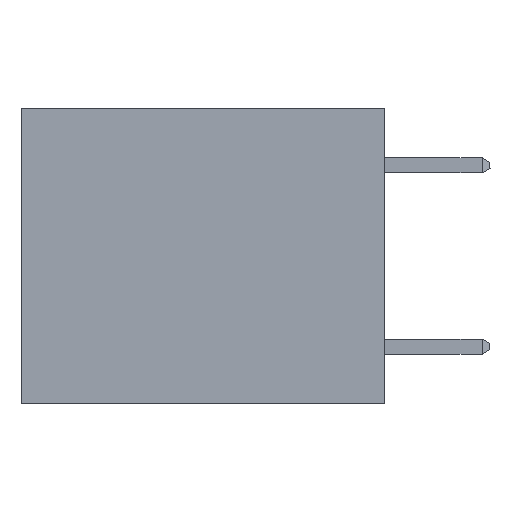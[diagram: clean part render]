
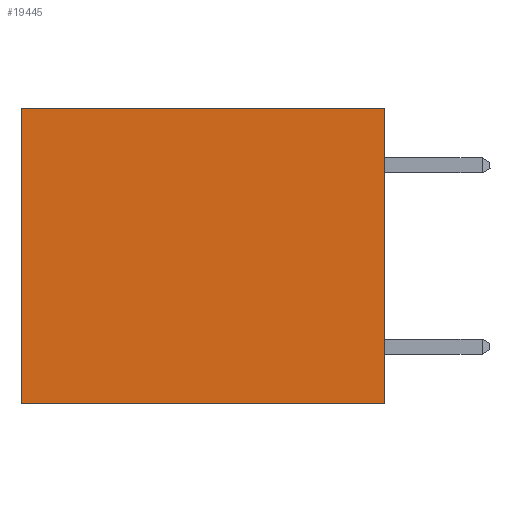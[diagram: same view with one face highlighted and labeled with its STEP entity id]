
A CAD part, left-side view. The second image highlights one B-rep face of the part: STEP entity #19445.
In plain terms, the highlighted planar face has unit normal (-1, 0, 0).
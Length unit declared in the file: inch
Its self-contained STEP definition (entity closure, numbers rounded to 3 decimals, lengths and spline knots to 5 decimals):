
#805 = VERTEX_POINT ( 'NONE', #16092 ) ;
#4127 = EDGE_CURVE ( 'NONE', #5492, #805, #22558, .T. ) ;
#5492 = VERTEX_POINT ( 'NONE', #27731 ) ;
#6005 = CARTESIAN_POINT ( 'NONE',  ( 0.3165, 0., -0.49 ) ) ;
#8502 = ORIENTED_EDGE ( 'NONE', *, *, #25466, .F. ) ;
#8824 = LINE ( 'NONE', #14661, #27597 ) ;
#9233 = VECTOR ( 'NONE', #26172, 39.37008 ) ;
#9883 = EDGE_CURVE ( 'NONE', #23448, #805, #23873, .T. ) ;
#10112 = VECTOR ( 'NONE', #18044, 39.37008 ) ;
#10651 = CARTESIAN_POINT ( 'NONE',  ( 0.3165, 0., -0.49 ) ) ;
#10740 = PLANE ( 'NONE',  #17032 ) ;
#11333 = LINE ( 'NONE', #6005, #9233 ) ;
#11965 = ORIENTED_EDGE ( 'NONE', *, *, #4127, .T. ) ;
#13971 = ORIENTED_EDGE ( 'NONE', *, *, #24392, .T. ) ;
#14238 = VERTEX_POINT ( 'NONE', #28294 ) ;
#14456 = CARTESIAN_POINT ( 'NONE',  ( 0.3165, 0., -0.49 ) ) ;
#14539 = ORIENTED_EDGE ( 'NONE', *, *, #9883, .F. ) ;
#14661 = CARTESIAN_POINT ( 'NONE',  ( 0.3165, 0., 0. ) ) ;
#14929 = DIRECTION ( 'NONE',  ( 0., 1., 0. ) ) ;
#16092 = CARTESIAN_POINT ( 'NONE',  ( 0.3165, 0.6, -0.49 ) ) ;
#17032 = AXIS2_PLACEMENT_3D ( 'NONE', #10651, #21950, #19601 ) ;
#17852 = CARTESIAN_POINT ( 'NONE',  ( 0.3165, 0.6, -0.49 ) ) ;
#18044 = DIRECTION ( 'NONE',  ( 0., 0., -1. ) ) ;
#19216 = EDGE_LOOP ( 'NONE', ( #11965, #14539, #8502, #13971 ) ) ;
#19377 = CARTESIAN_POINT ( 'NONE',  ( 0.3165, 0., -0.49 ) ) ;
#19445 = ADVANCED_FACE ( 'NONE', ( #25680 ), #10740, .F. ) ;
#19601 = DIRECTION ( 'NONE',  ( 0., 0., -1. ) ) ;
#21950 = DIRECTION ( 'NONE',  ( 1., 0., 0. ) ) ;
#22558 = LINE ( 'NONE', #17852, #10112 ) ;
#23448 = VERTEX_POINT ( 'NONE', #14456 ) ;
#23873 = LINE ( 'NONE', #19377, #28502 ) ;
#24392 = EDGE_CURVE ( 'NONE', #14238, #5492, #8824, .T. ) ;
#25466 = EDGE_CURVE ( 'NONE', #14238, #23448, #11333, .T. ) ;
#25680 = FACE_OUTER_BOUND ( 'NONE', #19216, .T. ) ;
#25931 = DIRECTION ( 'NONE',  ( 0., 1., 0. ) ) ;
#26172 = DIRECTION ( 'NONE',  ( 0., 0., -1. ) ) ;
#27597 = VECTOR ( 'NONE', #14929, 39.37008 ) ;
#27731 = CARTESIAN_POINT ( 'NONE',  ( 0.3165, 0.6, 0. ) ) ;
#28294 = CARTESIAN_POINT ( 'NONE',  ( 0.3165, 0., 0. ) ) ;
#28502 = VECTOR ( 'NONE', #25931, 39.37008 ) ;
